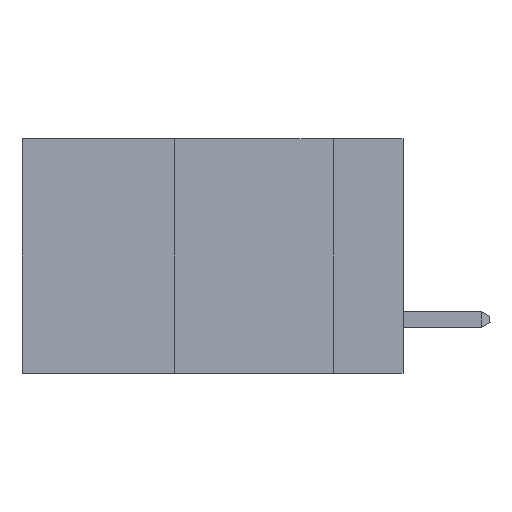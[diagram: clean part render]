
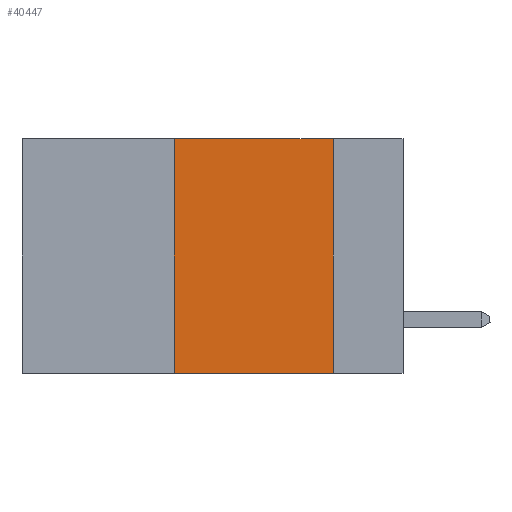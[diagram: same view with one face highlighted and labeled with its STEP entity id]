
A CAD part, left-side view. The second image highlights one B-rep face of the part: STEP entity #40447.
In plain terms, the highlighted planar face has unit normal (-1, 0, 0).
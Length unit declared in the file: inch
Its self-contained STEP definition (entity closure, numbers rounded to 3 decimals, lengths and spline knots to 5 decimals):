
#81 = VECTOR ( 'NONE', #39483, 39.37008 ) ;
#1954 = ORIENTED_EDGE ( 'NONE', *, *, #21317, .F. ) ;
#2060 = DIRECTION ( 'NONE',  ( 0., -1., 0. ) ) ;
#2693 = CARTESIAN_POINT ( 'NONE',  ( 0., 0.11, 0. ) ) ;
#4030 = DIRECTION ( 'NONE',  ( 0., 0., -1. ) ) ;
#8047 = VECTOR ( 'NONE', #2060, 39.37008 ) ;
#8102 = EDGE_CURVE ( 'NONE', #24124, #25635, #38694, .T. ) ;
#8215 = ORIENTED_EDGE ( 'NONE', *, *, #8102, .F. ) ;
#8483 = DIRECTION ( 'NONE',  ( 1., 0., 0. ) ) ;
#9705 = LINE ( 'NONE', #21167, #38797 ) ;
#10979 = AXIS2_PLACEMENT_3D ( 'NONE', #21100, #8483, #4030 ) ;
#12711 = LINE ( 'NONE', #33302, #81 ) ;
#14365 = PLANE ( 'NONE',  #10979 ) ;
#15383 = VERTEX_POINT ( 'NONE', #17753 ) ;
#17753 = CARTESIAN_POINT ( 'NONE',  ( 0., 0.36, -0.37 ) ) ;
#18878 = LINE ( 'NONE', #23074, #27400 ) ;
#21100 = CARTESIAN_POINT ( 'NONE',  ( 0., 0.6, 0. ) ) ;
#21167 = CARTESIAN_POINT ( 'NONE',  ( 0., 0.11, 0. ) ) ;
#21317 = EDGE_CURVE ( 'NONE', #25635, #29501, #9705, .T. ) ;
#21324 = CARTESIAN_POINT ( 'NONE',  ( 0., 0.6, 0. ) ) ;
#23074 = CARTESIAN_POINT ( 'NONE',  ( 0., 0.36, 0. ) ) ;
#23911 = EDGE_CURVE ( 'NONE', #15383, #29501, #12711, .T. ) ;
#24124 = VERTEX_POINT ( 'NONE', #28431 ) ;
#25635 = VERTEX_POINT ( 'NONE', #2693 ) ;
#26145 = FACE_OUTER_BOUND ( 'NONE', #35856, .T. ) ;
#26500 = ORIENTED_EDGE ( 'NONE', *, *, #28422, .F. ) ;
#27400 = VECTOR ( 'NONE', #36081, 39.37008 ) ;
#27487 = DIRECTION ( 'NONE',  ( 0., 0., -1. ) ) ;
#28422 = EDGE_CURVE ( 'NONE', #15383, #24124, #18878, .T. ) ;
#28431 = CARTESIAN_POINT ( 'NONE',  ( 0., 0.36, 0. ) ) ;
#29501 = VERTEX_POINT ( 'NONE', #33670 ) ;
#30960 = ORIENTED_EDGE ( 'NONE', *, *, #23911, .T. ) ;
#33302 = CARTESIAN_POINT ( 'NONE',  ( 0., 0.6, -0.37 ) ) ;
#33670 = CARTESIAN_POINT ( 'NONE',  ( 0., 0.11, -0.37 ) ) ;
#35856 = EDGE_LOOP ( 'NONE', ( #1954, #8215, #26500, #30960 ) ) ;
#36081 = DIRECTION ( 'NONE',  ( 0., 0., 1. ) ) ;
#38694 = LINE ( 'NONE', #21324, #8047 ) ;
#38797 = VECTOR ( 'NONE', #27487, 39.37008 ) ;
#39483 = DIRECTION ( 'NONE',  ( 0., -1., 0. ) ) ;
#40447 = ADVANCED_FACE ( 'NONE', ( #26145 ), #14365, .F. ) ;
